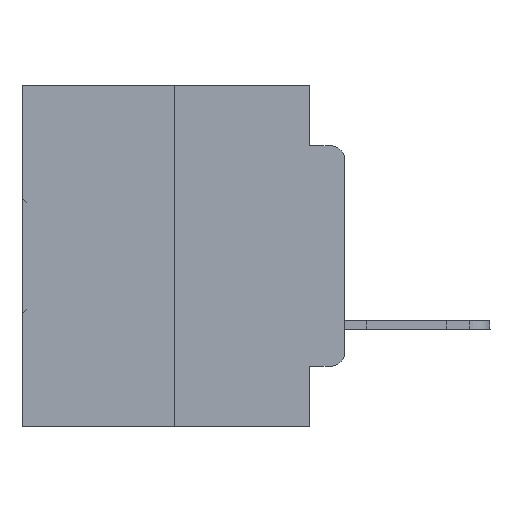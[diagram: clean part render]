
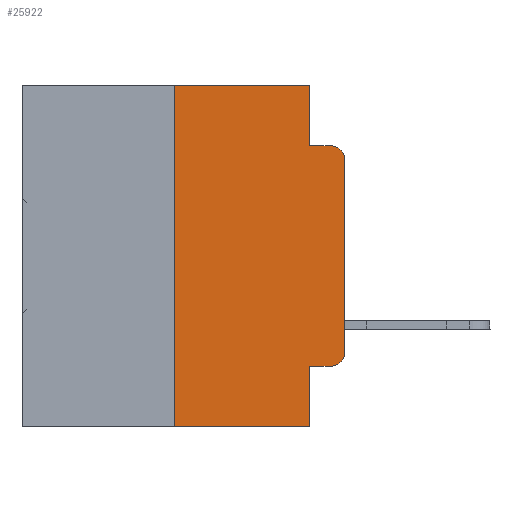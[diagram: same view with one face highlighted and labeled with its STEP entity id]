
A CAD part, left-side view. The second image highlights one B-rep face of the part: STEP entity #25922.
In plain terms, the highlighted planar face has unit normal (-1, 0, 0).
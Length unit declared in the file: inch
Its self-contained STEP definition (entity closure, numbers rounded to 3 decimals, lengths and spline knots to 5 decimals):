
#66 = VERTEX_POINT ( 'NONE', #14406 ) ;
#173 = VECTOR ( 'NONE', #23348, 39.37008 ) ;
#194 = ORIENTED_EDGE ( 'NONE', *, *, #16033, .F. ) ;
#346 = VERTEX_POINT ( 'NONE', #1730 ) ;
#444 = CARTESIAN_POINT ( 'NONE',  ( 0., 0.051, -0.0885 ) ) ;
#1041 = CIRCLE ( 'NONE', #31726, 0.02 ) ;
#1173 = CIRCLE ( 'NONE', #22352, 0.02 ) ;
#1730 = CARTESIAN_POINT ( 'NONE',  ( 0., 0.051, -0.4115 ) ) ;
#2397 = EDGE_CURVE ( 'NONE', #27392, #66, #11690, .T. ) ;
#2845 = AXIS2_PLACEMENT_3D ( 'NONE', #23823, #31296, #14181 ) ;
#2900 = CARTESIAN_POINT ( 'NONE',  ( 0., 0.051, 0. ) ) ;
#3441 = ORIENTED_EDGE ( 'NONE', *, *, #7422, .T. ) ;
#3909 = PLANE ( 'NONE',  #2845 ) ;
#4090 = DIRECTION ( 'NONE',  ( 0., 0., -1. ) ) ;
#4213 = EDGE_CURVE ( 'NONE', #30610, #26983, #1041, .T. ) ;
#4494 = ORIENTED_EDGE ( 'NONE', *, *, #26215, .F. ) ;
#5225 = LINE ( 'NONE', #2900, #6020 ) ;
#6020 = VECTOR ( 'NONE', #22812, 39.37008 ) ;
#6091 = VERTEX_POINT ( 'NONE', #444 ) ;
#6562 = DIRECTION ( 'NONE',  ( -1., 0., 0. ) ) ;
#6705 = ORIENTED_EDGE ( 'NONE', *, *, #18387, .F. ) ;
#6733 = CARTESIAN_POINT ( 'NONE',  ( 0., 0.02, -0.3915 ) ) ;
#7082 = DIRECTION ( 'NONE',  ( 0., 0., -1. ) ) ;
#7141 = ORIENTED_EDGE ( 'NONE', *, *, #22667, .T. ) ;
#7422 = EDGE_CURVE ( 'NONE', #15122, #30610, #29041, .T. ) ;
#7465 = DIRECTION ( 'NONE',  ( 0., -1., 0. ) ) ;
#7603 = CARTESIAN_POINT ( 'NONE',  ( 0., 0.02, -0.4115 ) ) ;
#7700 = VECTOR ( 'NONE', #13158, 39.37008 ) ;
#9671 = EDGE_CURVE ( 'NONE', #6091, #26983, #10736, .T. ) ;
#9981 = ORIENTED_EDGE ( 'NONE', *, *, #9671, .F. ) ;
#10715 = VECTOR ( 'NONE', #31450, 39.37008 ) ;
#10736 = LINE ( 'NONE', #30818, #173 ) ;
#10798 = DIRECTION ( 'NONE',  ( 0., -1., 0. ) ) ;
#10973 = CARTESIAN_POINT ( 'NONE',  ( 0., 0.25, -0.5 ) ) ;
#11273 = DIRECTION ( 'NONE',  ( 0., 0., 1. ) ) ;
#11690 = LINE ( 'NONE', #29458, #10715 ) ;
#11749 = VERTEX_POINT ( 'NONE', #32592 ) ;
#11759 = EDGE_CURVE ( 'NONE', #27392, #25053, #20627, .T. ) ;
#12383 = DIRECTION ( 'NONE',  ( -1., 0., 0. ) ) ;
#13158 = DIRECTION ( 'NONE',  ( 0., 0., 1. ) ) ;
#13621 = CARTESIAN_POINT ( 'NONE',  ( 0., 0.473, 0. ) ) ;
#14181 = DIRECTION ( 'NONE',  ( 0., 0., -1. ) ) ;
#14406 = CARTESIAN_POINT ( 'NONE',  ( 0., 0.051, -0.5 ) ) ;
#14972 = ORIENTED_EDGE ( 'NONE', *, *, #19132, .T. ) ;
#14985 = CARTESIAN_POINT ( 'NONE',  ( 0., 0.25, 0. ) ) ;
#15122 = VERTEX_POINT ( 'NONE', #16392 ) ;
#15399 = LINE ( 'NONE', #30522, #26405 ) ;
#16033 = EDGE_CURVE ( 'NONE', #25053, #11749, #26217, .T. ) ;
#16392 = CARTESIAN_POINT ( 'NONE',  ( 0., 0., -0.3915 ) ) ;
#16858 = CARTESIAN_POINT ( 'NONE',  ( 0., 0.02, -0.1085 ) ) ;
#17738 = EDGE_LOOP ( 'NONE', ( #3441, #22128, #9981, #4494, #194, #31533, #29150, #6705, #14972, #7141 ) ) ;
#18387 = EDGE_CURVE ( 'NONE', #346, #66, #26644, .T. ) ;
#18733 = CARTESIAN_POINT ( 'NONE',  ( 0., 0., 0. ) ) ;
#19132 = EDGE_CURVE ( 'NONE', #346, #31515, #15399, .T. ) ;
#20626 = VECTOR ( 'NONE', #32122, 39.37008 ) ;
#20627 = LINE ( 'NONE', #14985, #7700 ) ;
#21122 = CARTESIAN_POINT ( 'NONE',  ( 0., 0.25, 0. ) ) ;
#22083 = CARTESIAN_POINT ( 'NONE',  ( 0., 0.02, -0.0885 ) ) ;
#22128 = ORIENTED_EDGE ( 'NONE', *, *, #4213, .T. ) ;
#22352 = AXIS2_PLACEMENT_3D ( 'NONE', #6733, #6562, #4090 ) ;
#22667 = EDGE_CURVE ( 'NONE', #31515, #15122, #1173, .T. ) ;
#22812 = DIRECTION ( 'NONE',  ( 0., 0., -1. ) ) ;
#23348 = DIRECTION ( 'NONE',  ( 0., -1., 0. ) ) ;
#23823 = CARTESIAN_POINT ( 'NONE',  ( 0., 0.473, 0. ) ) ;
#24159 = CARTESIAN_POINT ( 'NONE',  ( 0., 0.051, 0. ) ) ;
#25053 = VERTEX_POINT ( 'NONE', #21122 ) ;
#25838 = CARTESIAN_POINT ( 'NONE',  ( 0., 0., -0.1085 ) ) ;
#25922 = ADVANCED_FACE ( 'NONE', ( #28971 ), #3909, .F. ) ;
#26215 = EDGE_CURVE ( 'NONE', #11749, #6091, #5225, .T. ) ;
#26217 = LINE ( 'NONE', #13621, #28486 ) ;
#26405 = VECTOR ( 'NONE', #7465, 39.37008 ) ;
#26644 = LINE ( 'NONE', #24159, #20626 ) ;
#26983 = VERTEX_POINT ( 'NONE', #22083 ) ;
#27392 = VERTEX_POINT ( 'NONE', #10973 ) ;
#27672 = VECTOR ( 'NONE', #11273, 39.37008 ) ;
#28486 = VECTOR ( 'NONE', #10798, 39.37008 ) ;
#28971 = FACE_OUTER_BOUND ( 'NONE', #17738, .T. ) ;
#29041 = LINE ( 'NONE', #18733, #27672 ) ;
#29150 = ORIENTED_EDGE ( 'NONE', *, *, #2397, .T. ) ;
#29458 = CARTESIAN_POINT ( 'NONE',  ( 0., 0.473, -0.5 ) ) ;
#30522 = CARTESIAN_POINT ( 'NONE',  ( 0., 0.051, -0.4115 ) ) ;
#30610 = VERTEX_POINT ( 'NONE', #25838 ) ;
#30818 = CARTESIAN_POINT ( 'NONE',  ( 0., 0.051, -0.0885 ) ) ;
#31296 = DIRECTION ( 'NONE',  ( 1., 0., 0. ) ) ;
#31450 = DIRECTION ( 'NONE',  ( 0., -1., 0. ) ) ;
#31515 = VERTEX_POINT ( 'NONE', #7603 ) ;
#31533 = ORIENTED_EDGE ( 'NONE', *, *, #11759, .F. ) ;
#31726 = AXIS2_PLACEMENT_3D ( 'NONE', #16858, #12383, #7082 ) ;
#32122 = DIRECTION ( 'NONE',  ( 0., 0., -1. ) ) ;
#32592 = CARTESIAN_POINT ( 'NONE',  ( 0., 0.051, 0. ) ) ;
